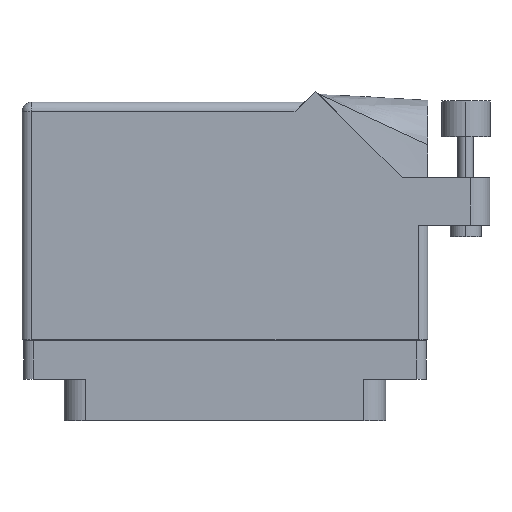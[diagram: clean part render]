
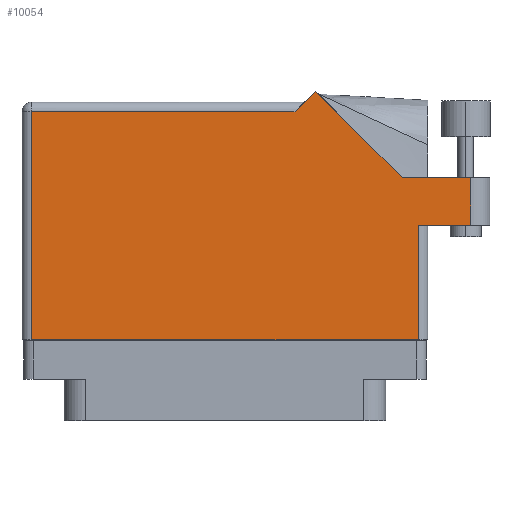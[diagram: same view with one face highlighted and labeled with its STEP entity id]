
A CAD part, front view. The second image highlights one B-rep face of the part: STEP entity #10054.
In plain terms, the highlighted face is planar.
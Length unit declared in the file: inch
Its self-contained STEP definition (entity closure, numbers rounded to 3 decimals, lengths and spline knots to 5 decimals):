
#293 = VECTOR ( 'NONE', #16580, 39.37008 ) ;
#2068 = CARTESIAN_POINT ( 'NONE',  ( 0.58371, 1.50071, 0.455 ) ) ;
#2079 = CARTESIAN_POINT ( 'NONE',  ( 1.706, 0.944, 0.455 ) ) ;
#2198 = DIRECTION ( 'NONE',  ( 0., 1., 0. ) ) ;
#2281 = CARTESIAN_POINT ( 'NONE',  ( -1.244, 1.368, 0.455 ) ) ;
#2913 = LINE ( 'NONE', #31966, #11291 ) ;
#3404 = VERTEX_POINT ( 'NONE', #2068 ) ;
#3721 = VECTOR ( 'NONE', #35825, 39.37008 ) ;
#4408 = CARTESIAN_POINT ( 'NONE',  ( 1.581, 0.637, 0.455 ) ) ;
#5641 = LINE ( 'NONE', #20411, #29393 ) ;
#5839 = CARTESIAN_POINT ( 'NONE',  ( 1.581, 0.944, 0.455 ) ) ;
#6928 = CARTESIAN_POINT ( 'NONE',  ( 1.14042, 0.944, 0.455 ) ) ;
#8478 = DIRECTION ( 'NONE',  ( -1., 0., 0. ) ) ;
#9782 = VECTOR ( 'NONE', #17826, 39.37008 ) ;
#10054 = ADVANCED_FACE ( 'NONE', ( #26155 ), #23006, .F. ) ;
#11291 = VECTOR ( 'NONE', #25177, 39.37008 ) ;
#12531 = CARTESIAN_POINT ( 'NONE',  ( 0.513, 1.43, 0.455 ) ) ;
#13637 = DIRECTION ( 'NONE',  ( 1., 0., 0. ) ) ;
#13671 = CARTESIAN_POINT ( 'NONE',  ( 1.244, 0.637, 0.455 ) ) ;
#14080 = DIRECTION ( 'NONE',  ( -1., 0., 0. ) ) ;
#14729 = VECTOR ( 'NONE', #33596, 39.37008 ) ;
#14774 = CARTESIAN_POINT ( 'NONE',  ( 0.451, 1.368, 0.455 ) ) ;
#15447 = VECTOR ( 'NONE', #2198, 39.37008 ) ;
#15631 = VERTEX_POINT ( 'NONE', #20647 ) ;
#15760 = DIRECTION ( 'NONE',  ( 0., 0., -1. ) ) ;
#15833 = VECTOR ( 'NONE', #38511, 39.37008 ) ;
#15956 = EDGE_CURVE ( 'NONE', #45888, #15631, #34871, .T. ) ;
#16002 = ORIENTED_EDGE ( 'NONE', *, *, #41947, .T. ) ;
#16189 = VERTEX_POINT ( 'NONE', #14774 ) ;
#16580 = DIRECTION ( 'NONE',  ( -0.707, 0.707, 0. ) ) ;
#17475 = LINE ( 'NONE', #32928, #41635 ) ;
#17826 = DIRECTION ( 'NONE',  ( -1., 0., 0. ) ) ;
#17966 = CARTESIAN_POINT ( 'NONE',  ( 1.244, -0.1, 0.455 ) ) ;
#19061 = ORIENTED_EDGE ( 'NONE', *, *, #28386, .T. ) ;
#19689 = ORIENTED_EDGE ( 'NONE', *, *, #22882, .T. ) ;
#20411 = CARTESIAN_POINT ( 'NONE',  ( 1.306, 0.637, 0.455 ) ) ;
#20647 = CARTESIAN_POINT ( 'NONE',  ( -1.244, -0.1, 0.455 ) ) ;
#21364 = EDGE_CURVE ( 'NONE', #15631, #36245, #39947, .T. ) ;
#22388 = ORIENTED_EDGE ( 'NONE', *, *, #31353, .T. ) ;
#22882 = EDGE_CURVE ( 'NONE', #45919, #35935, #5641, .T. ) ;
#23006 = PLANE ( 'NONE',  #37084 ) ;
#23334 = LINE ( 'NONE', #34952, #293 ) ;
#23412 = LINE ( 'NONE', #12531, #14729 ) ;
#24612 = EDGE_LOOP ( 'NONE', ( #19689, #22388, #19061, #27360, #16002, #42272, #27591, #33512, #38806 ) ) ;
#25177 = DIRECTION ( 'NONE',  ( 0., 1., 0. ) ) ;
#26155 = FACE_OUTER_BOUND ( 'NONE', #24612, .T. ) ;
#27360 = ORIENTED_EDGE ( 'NONE', *, *, #47371, .T. ) ;
#27560 = EDGE_CURVE ( 'NONE', #36245, #45919, #2913, .T. ) ;
#27591 = ORIENTED_EDGE ( 'NONE', *, *, #15956, .T. ) ;
#28386 = EDGE_CURVE ( 'NONE', #47263, #39544, #43476, .T. ) ;
#29266 = CARTESIAN_POINT ( 'NONE',  ( -1.306, -0.1, 0.455 ) ) ;
#29393 = VECTOR ( 'NONE', #13637, 39.37008 ) ;
#30508 = CARTESIAN_POINT ( 'NONE',  ( -1.244, -0.1, 0.455 ) ) ;
#31353 = EDGE_CURVE ( 'NONE', #35935, #47263, #43356, .T. ) ;
#31966 = CARTESIAN_POINT ( 'NONE',  ( 1.244, 0.637, 0.455 ) ) ;
#32928 = CARTESIAN_POINT ( 'NONE',  ( -1.306, 1.368, 0.455 ) ) ;
#33512 = ORIENTED_EDGE ( 'NONE', *, *, #21364, .T. ) ;
#33596 = DIRECTION ( 'NONE',  ( -0.707, -0.707, 0. ) ) ;
#33749 = CARTESIAN_POINT ( 'NONE',  ( 1.581, 0.944, 0.455 ) ) ;
#34871 = LINE ( 'NONE', #30508, #15833 ) ;
#34952 = CARTESIAN_POINT ( 'NONE',  ( 1.14042, 0.944, 0.455 ) ) ;
#35825 = DIRECTION ( 'NONE',  ( 1., 0., 0. ) ) ;
#35935 = VERTEX_POINT ( 'NONE', #4408 ) ;
#36245 = VERTEX_POINT ( 'NONE', #17966 ) ;
#37084 = AXIS2_PLACEMENT_3D ( 'NONE', #37779, #15760, #8478 ) ;
#37779 = CARTESIAN_POINT ( 'NONE',  ( -1.306, 1.43, 0.455 ) ) ;
#38511 = DIRECTION ( 'NONE',  ( 0., -1., 0. ) ) ;
#38674 = EDGE_CURVE ( 'NONE', #16189, #45888, #17475, .T. ) ;
#38806 = ORIENTED_EDGE ( 'NONE', *, *, #27560, .T. ) ;
#39544 = VERTEX_POINT ( 'NONE', #6928 ) ;
#39947 = LINE ( 'NONE', #29266, #3721 ) ;
#41635 = VECTOR ( 'NONE', #14080, 39.37008 ) ;
#41947 = EDGE_CURVE ( 'NONE', #3404, #16189, #23412, .T. ) ;
#42272 = ORIENTED_EDGE ( 'NONE', *, *, #38674, .T. ) ;
#43356 = LINE ( 'NONE', #5839, #15447 ) ;
#43476 = LINE ( 'NONE', #2079, #9782 ) ;
#45888 = VERTEX_POINT ( 'NONE', #2281 ) ;
#45919 = VERTEX_POINT ( 'NONE', #13671 ) ;
#47263 = VERTEX_POINT ( 'NONE', #33749 ) ;
#47371 = EDGE_CURVE ( 'NONE', #39544, #3404, #23334, .T. ) ;
